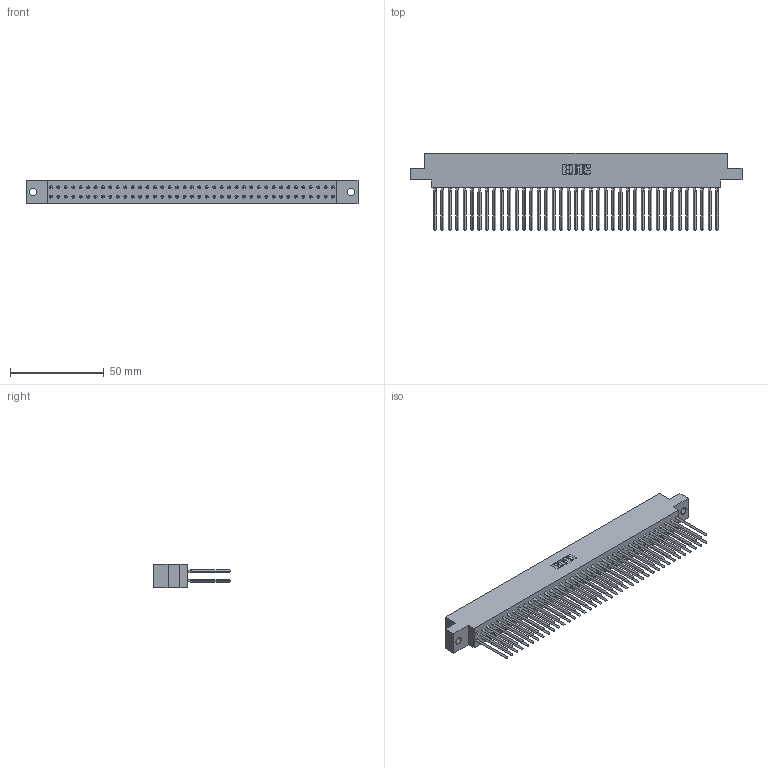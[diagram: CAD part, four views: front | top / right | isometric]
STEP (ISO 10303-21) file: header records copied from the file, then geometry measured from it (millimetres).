
FILE_DESCRIPTION (( 'STEP AP203' ), '1' );
FILE_NAME ('317-078-543-804.STEP', '2020-02-28T08:59:03', ( '' ), ( '' ), 'SwSTEP 2.0', 'SolidWorks 2016', '' );
FILE_SCHEMA (( 'CONFIG_CONTROL_DESIGN' ));
Length unit declared in the file: inch
Products named in the file (3): 317 Part_.156 Dia - TH; 317-078-543-804; 317-290-001_543
Assembly tree (79 placements, depth 2):
  317-078-543-804
    317 Part_.156 Dia - TH
    317-290-001_543  x78
Bounding box: 177.24 x 41.15 x 12.7 mm (x, y, z)
Volume: 29945.5 mm3; surface area: 45137.7 mm2
Topology: 79 solids, 79 shells, 7044 faces, 19541 edges, 12584 vertices
Faces by surface type: plane 5752, cylinder 980, bspline 312
Entity records: 56796 total; most frequent: CARTESIAN_POINT 10323, ORIENTED_EDGE 9822, DIRECTION 8193, EDGE_CURVE 4911, VECTOR 4655, LINE 4655, VERTEX_POINT 3267, AXIS2_PLACEMENT_3D 1769
